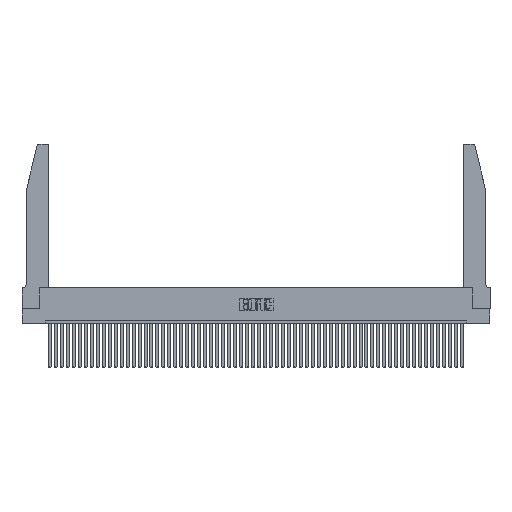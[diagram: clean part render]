
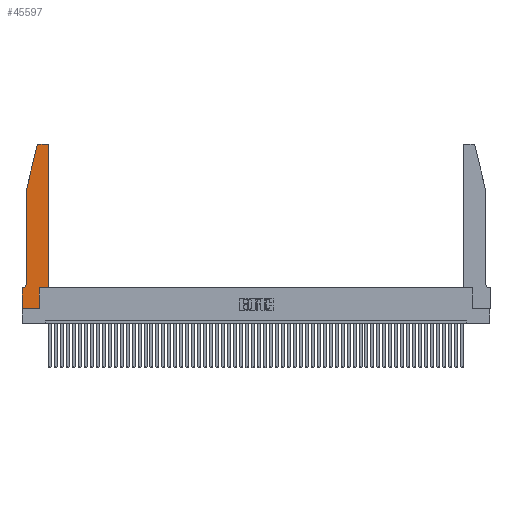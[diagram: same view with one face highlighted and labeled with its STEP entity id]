
A CAD part, top view. The second image highlights one B-rep face of the part: STEP entity #45597.
In plain terms, the highlighted planar face has unit normal (0, 0, 1).
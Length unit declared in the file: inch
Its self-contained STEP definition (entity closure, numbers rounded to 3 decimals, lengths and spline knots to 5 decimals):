
#43 = VERTEX_POINT ( 'NONE', #44611 ) ;
#216 = EDGE_CURVE ( 'NONE', #41851, #26964, #5455, .T. ) ;
#278 = VERTEX_POINT ( 'NONE', #46940 ) ;
#994 = CARTESIAN_POINT ( 'NONE',  ( 0., 0., 0.37 ) ) ;
#1765 = CARTESIAN_POINT ( 'NONE',  ( 0.284, 2.75, 0.37 ) ) ;
#1814 = AXIS2_PLACEMENT_3D ( 'NONE', #26294, #34993, #23445 ) ;
#2202 = CARTESIAN_POINT ( 'NONE',  ( 0.4205, 2.72, 0.37 ) ) ;
#2741 = LINE ( 'NONE', #994, #5278 ) ;
#3257 = CIRCLE ( 'NONE', #40007, 0.07 ) ;
#3300 = VERTEX_POINT ( 'NONE', #43203 ) ;
#3784 = DIRECTION ( 'NONE',  ( 0., 1., 0. ) ) ;
#5119 = CARTESIAN_POINT ( 'NONE',  ( 0.0755, 0.35, 0.37 ) ) ;
#5278 = VECTOR ( 'NONE', #9433, 39.37008 ) ;
#5455 = CIRCLE ( 'NONE', #1814, 0.03 ) ;
#5586 = CARTESIAN_POINT ( 'NONE',  ( 0., 0., 0.37 ) ) ;
#6063 = EDGE_CURVE ( 'NONE', #18474, #19978, #44388, .T. ) ;
#6140 = ORIENTED_EDGE ( 'NONE', *, *, #216, .T. ) ;
#6201 = ORIENTED_EDGE ( 'NONE', *, *, #33960, .T. ) ;
#6631 = CARTESIAN_POINT ( 'NONE',  ( 0.4505, 0.35, 0.37 ) ) ;
#6969 = CARTESIAN_POINT ( 'NONE',  ( 0.0755, 2., 0.37 ) ) ;
#7586 = CARTESIAN_POINT ( 'NONE',  ( 0., 0.35, 0.37 ) ) ;
#8491 = EDGE_CURVE ( 'NONE', #38013, #42570, #22693, .T. ) ;
#8858 = ORIENTED_EDGE ( 'NONE', *, *, #30294, .T. ) ;
#9433 = DIRECTION ( 'NONE',  ( 1., 0., 0. ) ) ;
#9599 = EDGE_CURVE ( 'NONE', #43, #3300, #46457, .T. ) ;
#9814 = CARTESIAN_POINT ( 'NONE',  ( 0.25487, 2.72718, 0.37 ) ) ;
#10906 = EDGE_CURVE ( 'NONE', #278, #40735, #23598, .T. ) ;
#12140 = ORIENTED_EDGE ( 'NONE', *, *, #10906, .T. ) ;
#12892 = EDGE_LOOP ( 'NONE', ( #6201, #6140, #13101, #43487, #8858, #47682, #42617, #45481, #35632, #46690, #34493, #12140 ) ) ;
#13101 = ORIENTED_EDGE ( 'NONE', *, *, #38386, .T. ) ;
#13311 = EDGE_CURVE ( 'NONE', #30757, #278, #37439, .T. ) ;
#13455 = DIRECTION ( 'NONE',  ( -1., 0., 0. ) ) ;
#13989 = VECTOR ( 'NONE', #20871, 39.37008 ) ;
#16282 = CARTESIAN_POINT ( 'NONE',  ( 0.0755, 2., 0.37 ) ) ;
#16659 = CARTESIAN_POINT ( 'NONE',  ( 0.2865, 0.35, 0.37 ) ) ;
#17492 = EDGE_CURVE ( 'NONE', #3300, #30757, #32672, .T. ) ;
#18089 = CARTESIAN_POINT ( 'NONE',  ( 0., 0.35, 0.37 ) ) ;
#18474 = VERTEX_POINT ( 'NONE', #18089 ) ;
#18794 = CARTESIAN_POINT ( 'NONE',  ( 0.0755, 2., 0.37 ) ) ;
#19665 = VECTOR ( 'NONE', #31043, 39.37008 ) ;
#19978 = VERTEX_POINT ( 'NONE', #5586 ) ;
#20278 = EDGE_CURVE ( 'NONE', #19978, #43, #2741, .T. ) ;
#20871 = DIRECTION ( 'NONE',  ( 0., -1., 0. ) ) ;
#21139 = FACE_OUTER_BOUND ( 'NONE', #12892, .T. ) ;
#21799 = CARTESIAN_POINT ( 'NONE',  ( 0.4505, 0.35, 0.37 ) ) ;
#22693 = LINE ( 'NONE', #6969, #49872 ) ;
#23445 = DIRECTION ( 'NONE',  ( 1., 0., 0. ) ) ;
#23598 = CIRCLE ( 'NONE', #45377, 0.03 ) ;
#25287 = DIRECTION ( 'NONE',  ( -1., 0., 0. ) ) ;
#25458 = DIRECTION ( 'NONE',  ( 0., 0., -1. ) ) ;
#26294 = CARTESIAN_POINT ( 'NONE',  ( 0.284, 2.72, 0.37 ) ) ;
#26398 = VECTOR ( 'NONE', #39498, 39.37008 ) ;
#26561 = CARTESIAN_POINT ( 'NONE',  ( 0.4505, 0.35, 0.37 ) ) ;
#26964 = VERTEX_POINT ( 'NONE', #9814 ) ;
#27286 = VECTOR ( 'NONE', #47668, 39.37008 ) ;
#30068 = CARTESIAN_POINT ( 'NONE',  ( 0.0055, 0.35, 0.37 ) ) ;
#30294 = EDGE_CURVE ( 'NONE', #42570, #45442, #3257, .T. ) ;
#30591 = CARTESIAN_POINT ( 'NONE',  ( 0.4205, 2.75, 0.37 ) ) ;
#30757 = VERTEX_POINT ( 'NONE', #6631 ) ;
#31043 = DIRECTION ( 'NONE',  ( -1., 0., 0. ) ) ;
#32613 = EDGE_CURVE ( 'NONE', #45442, #18474, #52064, .T. ) ;
#32672 = LINE ( 'NONE', #26561, #41708 ) ;
#33960 = EDGE_CURVE ( 'NONE', #40735, #41851, #36409, .T. ) ;
#34493 = ORIENTED_EDGE ( 'NONE', *, *, #13311, .T. ) ;
#34993 = DIRECTION ( 'NONE',  ( 0., 0., 1. ) ) ;
#35632 = ORIENTED_EDGE ( 'NONE', *, *, #9599, .T. ) ;
#36409 = LINE ( 'NONE', #42079, #19665 ) ;
#36998 = DIRECTION ( 'NONE',  ( 1., 0., 0. ) ) ;
#37439 = LINE ( 'NONE', #21799, #49770 ) ;
#38013 = VERTEX_POINT ( 'NONE', #16282 ) ;
#38386 = EDGE_CURVE ( 'NONE', #26964, #38013, #48572, .T. ) ;
#39498 = DIRECTION ( 'NONE',  ( 0., 1., 0. ) ) ;
#40007 = AXIS2_PLACEMENT_3D ( 'NONE', #45937, #25458, #25287 ) ;
#40322 = DIRECTION ( 'NONE',  ( 1., 0., 0. ) ) ;
#40735 = VERTEX_POINT ( 'NONE', #30591 ) ;
#41145 = DIRECTION ( 'NONE',  ( 0., 0., 1. ) ) ;
#41708 = VECTOR ( 'NONE', #40322, 39.37008 ) ;
#41851 = VERTEX_POINT ( 'NONE', #1765 ) ;
#42079 = CARTESIAN_POINT ( 'NONE',  ( 0.2605, 2.75, 0.37 ) ) ;
#42570 = VERTEX_POINT ( 'NONE', #51204 ) ;
#42617 = ORIENTED_EDGE ( 'NONE', *, *, #6063, .T. ) ;
#42769 = AXIS2_PLACEMENT_3D ( 'NONE', #7586, #41145, #36998 ) ;
#43203 = CARTESIAN_POINT ( 'NONE',  ( 0.2865, 0.35, 0.37 ) ) ;
#43365 = DIRECTION ( 'NONE',  ( 0., 0., 1. ) ) ;
#43487 = ORIENTED_EDGE ( 'NONE', *, *, #8491, .T. ) ;
#44013 = DIRECTION ( 'NONE',  ( 0., -1., 0. ) ) ;
#44388 = LINE ( 'NONE', #49074, #13989 ) ;
#44611 = CARTESIAN_POINT ( 'NONE',  ( 0.2865, 0., 0.37 ) ) ;
#45377 = AXIS2_PLACEMENT_3D ( 'NONE', #2202, #43365, #50912 ) ;
#45442 = VERTEX_POINT ( 'NONE', #30068 ) ;
#45481 = ORIENTED_EDGE ( 'NONE', *, *, #20278, .T. ) ;
#45597 = ADVANCED_FACE ( 'NONE', ( #21139 ), #53115, .T. ) ;
#45937 = CARTESIAN_POINT ( 'NONE',  ( 0.0055, 0.42, 0.37 ) ) ;
#46241 = VECTOR ( 'NONE', #13455, 39.37008 ) ;
#46457 = LINE ( 'NONE', #16659, #26398 ) ;
#46690 = ORIENTED_EDGE ( 'NONE', *, *, #17492, .T. ) ;
#46940 = CARTESIAN_POINT ( 'NONE',  ( 0.4505, 2.72, 0.37 ) ) ;
#47668 = DIRECTION ( 'NONE',  ( -0.239, -0.971, 0. ) ) ;
#47682 = ORIENTED_EDGE ( 'NONE', *, *, #32613, .T. ) ;
#48572 = LINE ( 'NONE', #18794, #27286 ) ;
#49074 = CARTESIAN_POINT ( 'NONE',  ( 0., 0., 0.37 ) ) ;
#49770 = VECTOR ( 'NONE', #3784, 39.37008 ) ;
#49872 = VECTOR ( 'NONE', #44013, 39.37008 ) ;
#50912 = DIRECTION ( 'NONE',  ( 1., 0., 0. ) ) ;
#51204 = CARTESIAN_POINT ( 'NONE',  ( 0.0755, 0.42, 0.37 ) ) ;
#52064 = LINE ( 'NONE', #5119, #46241 ) ;
#53115 = PLANE ( 'NONE',  #42769 ) ;
